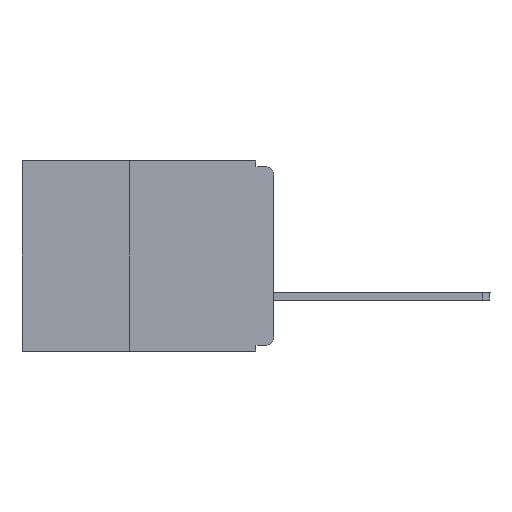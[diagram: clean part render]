
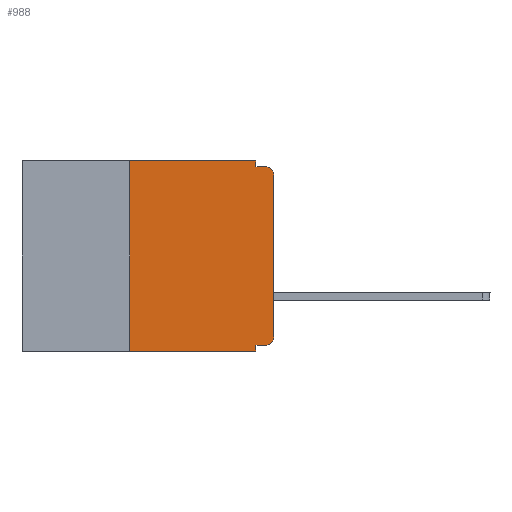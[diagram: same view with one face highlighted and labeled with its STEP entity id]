
A CAD part, left-side view. The second image highlights one B-rep face of the part: STEP entity #988.
In plain terms, the highlighted planar face has unit normal (-1, 0, 0).
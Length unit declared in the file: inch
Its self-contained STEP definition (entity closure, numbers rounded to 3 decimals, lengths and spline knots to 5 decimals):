
#84 = ORIENTED_EDGE ( 'NONE', *, *, #9473, .T. ) ;
#89 = DIRECTION ( 'NONE',  ( 0., 0., -1. ) ) ;
#198 = DIRECTION ( 'NONE',  ( 0., 0., 1. ) ) ;
#264 = VERTEX_POINT ( 'NONE', #4945 ) ;
#510 = ORIENTED_EDGE ( 'NONE', *, *, #8638, .T. ) ;
#940 = LINE ( 'NONE', #1972, #2641 ) ;
#988 = ADVANCED_FACE ( 'NONE', ( #5949 ), #9646, .F. ) ;
#1522 = DIRECTION ( 'NONE',  ( 0., -1., 0. ) ) ;
#1676 = DIRECTION ( 'NONE',  ( 0., 0., -1. ) ) ;
#1779 = ORIENTED_EDGE ( 'NONE', *, *, #5259, .T. ) ;
#1838 = CARTESIAN_POINT ( 'NONE',  ( 0., 0.031, 0. ) ) ;
#1916 = ORIENTED_EDGE ( 'NONE', *, *, #4301, .F. ) ;
#1972 = CARTESIAN_POINT ( 'NONE',  ( 0., 0.031, -0.33 ) ) ;
#2005 = LINE ( 'NONE', #5219, #6197 ) ;
#2076 = VECTOR ( 'NONE', #6398, 39.37008 ) ;
#2160 = ORIENTED_EDGE ( 'NONE', *, *, #9301, .T. ) ;
#2192 = LINE ( 'NONE', #10670, #10554 ) ;
#2499 = CARTESIAN_POINT ( 'NONE',  ( 0., 0.25, 0. ) ) ;
#2501 = CARTESIAN_POINT ( 'NONE',  ( 0., 0.015, -0.025 ) ) ;
#2641 = VECTOR ( 'NONE', #6287, 39.37008 ) ;
#2923 = CARTESIAN_POINT ( 'NONE',  ( 0., 0.437, 0. ) ) ;
#3058 = DIRECTION ( 'NONE',  ( 0., -1., 0. ) ) ;
#3071 = CARTESIAN_POINT ( 'NONE',  ( 0., 0.25, -0.33 ) ) ;
#3134 = CARTESIAN_POINT ( 'NONE',  ( 0., 0., -0.01 ) ) ;
#3209 = VECTOR ( 'NONE', #5728, 39.37008 ) ;
#3450 = LINE ( 'NONE', #1838, #5299 ) ;
#3570 = CIRCLE ( 'NONE', #8418, 0.015 ) ;
#3662 = CARTESIAN_POINT ( 'NONE',  ( 0., 0.031, -0.32 ) ) ;
#3773 = AXIS2_PLACEMENT_3D ( 'NONE', #2923, #8665, #10438 ) ;
#3808 = VECTOR ( 'NONE', #3058, 39.37008 ) ;
#3888 = EDGE_CURVE ( 'NONE', #5947, #10441, #7972, .T. ) ;
#4158 = ORIENTED_EDGE ( 'NONE', *, *, #10238, .F. ) ;
#4282 = CIRCLE ( 'NONE', #10707, 0.015 ) ;
#4301 = EDGE_CURVE ( 'NONE', #10441, #264, #2192, .T. ) ;
#4453 = EDGE_LOOP ( 'NONE', ( #2160, #510, #4158, #8169, #1916, #5980, #1779, #6168, #9714, #84 ) ) ;
#4621 = CARTESIAN_POINT ( 'NONE',  ( 0., 0., -0.305 ) ) ;
#4708 = CARTESIAN_POINT ( 'NONE',  ( 0., 0.25, -0.33 ) ) ;
#4855 = CARTESIAN_POINT ( 'NONE',  ( 0., 0.031, -0.01 ) ) ;
#4945 = CARTESIAN_POINT ( 'NONE',  ( 0., 0.031, 0. ) ) ;
#5029 = CARTESIAN_POINT ( 'NONE',  ( 0., 0.015, -0.32 ) ) ;
#5194 = VECTOR ( 'NONE', #1522, 39.37008 ) ;
#5219 = CARTESIAN_POINT ( 'NONE',  ( 0., 0., 0. ) ) ;
#5259 = EDGE_CURVE ( 'NONE', #5947, #8662, #10131, .T. ) ;
#5265 = CARTESIAN_POINT ( 'NONE',  ( 0., 0.015, -0.01 ) ) ;
#5299 = VECTOR ( 'NONE', #89, 39.37008 ) ;
#5358 = CARTESIAN_POINT ( 'NONE',  ( 0., 0.015, -0.305 ) ) ;
#5398 = LINE ( 'NONE', #3134, #3808 ) ;
#5728 = DIRECTION ( 'NONE',  ( 0., 1., 0. ) ) ;
#5947 = VERTEX_POINT ( 'NONE', #3071 ) ;
#5949 = FACE_OUTER_BOUND ( 'NONE', #4453, .T. ) ;
#5980 = ORIENTED_EDGE ( 'NONE', *, *, #3888, .F. ) ;
#6043 = EDGE_CURVE ( 'NONE', #7544, #9392, #9370, .T. ) ;
#6168 = ORIENTED_EDGE ( 'NONE', *, *, #10086, .F. ) ;
#6197 = VECTOR ( 'NONE', #198, 39.37008 ) ;
#6229 = DIRECTION ( 'NONE',  ( -1., 0., 0. ) ) ;
#6273 = VERTEX_POINT ( 'NONE', #5265 ) ;
#6287 = DIRECTION ( 'NONE',  ( 0., 0., -1. ) ) ;
#6398 = DIRECTION ( 'NONE',  ( 0., 0., 1. ) ) ;
#6448 = CARTESIAN_POINT ( 'NONE',  ( 0., 0., -0.025 ) ) ;
#6538 = CARTESIAN_POINT ( 'NONE',  ( 0., 0.437, -0.33 ) ) ;
#6756 = DIRECTION ( 'NONE',  ( -1., 0., 0. ) ) ;
#7070 = DIRECTION ( 'NONE',  ( 0., 0., -1. ) ) ;
#7308 = DIRECTION ( 'NONE',  ( 0., -1., 0. ) ) ;
#7422 = EDGE_CURVE ( 'NONE', #264, #8548, #3450, .T. ) ;
#7544 = VERTEX_POINT ( 'NONE', #5029 ) ;
#7681 = CARTESIAN_POINT ( 'NONE',  ( 0., 0.031, -0.33 ) ) ;
#7972 = LINE ( 'NONE', #4708, #2076 ) ;
#8160 = CARTESIAN_POINT ( 'NONE',  ( 0., 0., -0.32 ) ) ;
#8169 = ORIENTED_EDGE ( 'NONE', *, *, #7422, .F. ) ;
#8361 = VERTEX_POINT ( 'NONE', #6448 ) ;
#8418 = AXIS2_PLACEMENT_3D ( 'NONE', #5358, #6229, #7070 ) ;
#8548 = VERTEX_POINT ( 'NONE', #4855 ) ;
#8638 = EDGE_CURVE ( 'NONE', #8361, #6273, #4282, .T. ) ;
#8662 = VERTEX_POINT ( 'NONE', #7681 ) ;
#8665 = DIRECTION ( 'NONE',  ( 1., 0., 0. ) ) ;
#9301 = EDGE_CURVE ( 'NONE', #10750, #8361, #2005, .T. ) ;
#9370 = LINE ( 'NONE', #8160, #3209 ) ;
#9392 = VERTEX_POINT ( 'NONE', #3662 ) ;
#9473 = EDGE_CURVE ( 'NONE', #7544, #10750, #3570, .T. ) ;
#9646 = PLANE ( 'NONE',  #3773 ) ;
#9714 = ORIENTED_EDGE ( 'NONE', *, *, #6043, .F. ) ;
#10086 = EDGE_CURVE ( 'NONE', #9392, #8662, #940, .T. ) ;
#10131 = LINE ( 'NONE', #6538, #5194 ) ;
#10238 = EDGE_CURVE ( 'NONE', #8548, #6273, #5398, .T. ) ;
#10438 = DIRECTION ( 'NONE',  ( 0., 0., -1. ) ) ;
#10441 = VERTEX_POINT ( 'NONE', #2499 ) ;
#10554 = VECTOR ( 'NONE', #7308, 39.37008 ) ;
#10670 = CARTESIAN_POINT ( 'NONE',  ( 0., 0.437, 0. ) ) ;
#10707 = AXIS2_PLACEMENT_3D ( 'NONE', #2501, #6756, #1676 ) ;
#10750 = VERTEX_POINT ( 'NONE', #4621 ) ;
